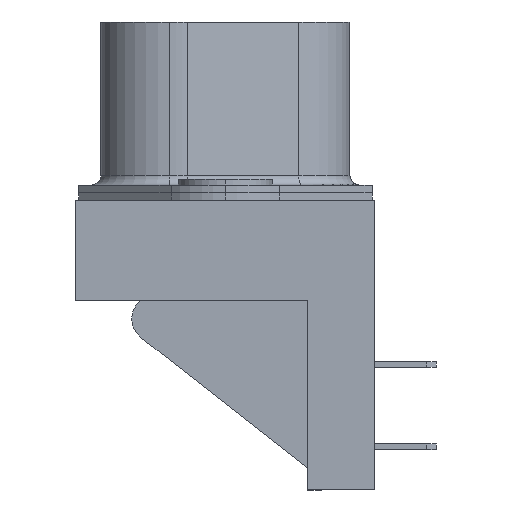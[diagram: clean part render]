
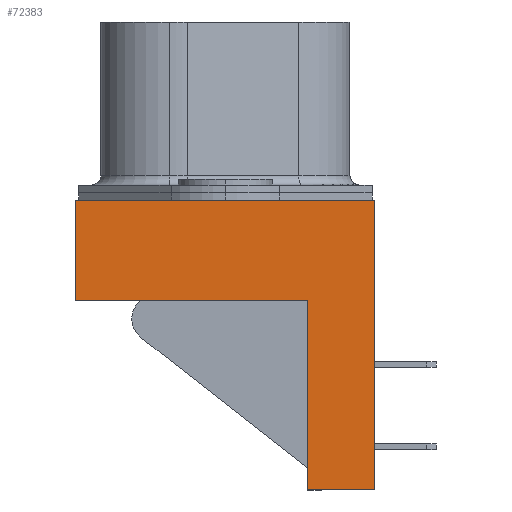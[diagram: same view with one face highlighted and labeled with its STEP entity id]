
A CAD part, left-side view. The second image highlights one B-rep face of the part: STEP entity #72383.
In plain terms, the highlighted planar face has unit normal (-1, 0, 0).
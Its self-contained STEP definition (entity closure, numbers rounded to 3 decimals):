
#6338 = VECTOR ( 'NONE', #7277, 1000. ) ;
#7079 = LINE ( 'NONE', #116483, #112464 ) ;
#7277 = DIRECTION ( 'NONE',  ( 0., 1., 0. ) ) ;
#9020 = CARTESIAN_POINT ( 'NONE',  ( -4.125, 7.8, -5.2 ) ) ;
#9100 = CARTESIAN_POINT ( 'NONE',  ( -4.125, 7.8, -15.1 ) ) ;
#12215 = ORIENTED_EDGE ( 'NONE', *, *, #30796, .T. ) ;
#16595 = EDGE_CURVE ( 'NONE', #127421, #80010, #158144, .T. ) ;
#17014 = AXIS2_PLACEMENT_3D ( 'NONE', #9100, #148927, #162362 ) ;
#20679 = CARTESIAN_POINT ( 'NONE',  ( -4.125, -7.8, -15.1 ) ) ;
#30796 = EDGE_CURVE ( 'NONE', #80010, #71657, #39707, .T. ) ;
#39707 = LINE ( 'NONE', #149103, #87490 ) ;
#47258 = DIRECTION ( 'NONE',  ( 0., 0., 1. ) ) ;
#51379 = DIRECTION ( 'NONE',  ( 0., 0., 1. ) ) ;
#57120 = EDGE_CURVE ( 'NONE', #147995, #71657, #125029, .T. ) ;
#58503 = VERTEX_POINT ( 'NONE', #109397 ) ;
#63355 = LINE ( 'NONE', #144104, #88697 ) ;
#64720 = VECTOR ( 'NONE', #99892, 1000. ) ;
#64874 = EDGE_CURVE ( 'NONE', #58503, #126019, #130157, .T. ) ;
#65377 = EDGE_CURVE ( 'NONE', #127421, #58503, #7079, .T. ) ;
#71657 = VERTEX_POINT ( 'NONE', #162786 ) ;
#72383 = ADVANCED_FACE ( 'NONE', ( #74632 ), #129359, .T. ) ;
#74632 = FACE_OUTER_BOUND ( 'NONE', #95636, .T. ) ;
#76342 = CARTESIAN_POINT ( 'NONE',  ( -4.125, 7.8, -5.2 ) ) ;
#80010 = VERTEX_POINT ( 'NONE', #20679 ) ;
#87490 = VECTOR ( 'NONE', #51379, 1000. ) ;
#88697 = VECTOR ( 'NONE', #47258, 1000. ) ;
#89996 = DIRECTION ( 'NONE',  ( 0., -1., 0. ) ) ;
#90868 = CARTESIAN_POINT ( 'NONE',  ( -4.125, 7.8, -15.1 ) ) ;
#93378 = EDGE_CURVE ( 'NONE', #126019, #147995, #63355, .T. ) ;
#95636 = EDGE_LOOP ( 'NONE', ( #129250, #99727, #172409, #12215, #135933, #114596 ) ) ;
#99727 = ORIENTED_EDGE ( 'NONE', *, *, #65377, .F. ) ;
#99892 = DIRECTION ( 'NONE',  ( 0., -1., 0. ) ) ;
#101210 = CARTESIAN_POINT ( 'NONE',  ( -4.125, 7.8, 0. ) ) ;
#109397 = CARTESIAN_POINT ( 'NONE',  ( -4.125, -4.3, -5.2 ) ) ;
#112464 = VECTOR ( 'NONE', #171159, 1000. ) ;
#114596 = ORIENTED_EDGE ( 'NONE', *, *, #93378, .F. ) ;
#116483 = CARTESIAN_POINT ( 'NONE',  ( -4.125, -4.3, -15.1 ) ) ;
#125029 = LINE ( 'NONE', #126829, #64720 ) ;
#126019 = VERTEX_POINT ( 'NONE', #76342 ) ;
#126829 = CARTESIAN_POINT ( 'NONE',  ( -4.125, 7.8, 0. ) ) ;
#127421 = VERTEX_POINT ( 'NONE', #143455 ) ;
#129250 = ORIENTED_EDGE ( 'NONE', *, *, #64874, .F. ) ;
#129359 = PLANE ( 'NONE',  #17014 ) ;
#130157 = LINE ( 'NONE', #9020, #6338 ) ;
#135933 = ORIENTED_EDGE ( 'NONE', *, *, #57120, .F. ) ;
#143455 = CARTESIAN_POINT ( 'NONE',  ( -4.125, -4.3, -15.1 ) ) ;
#144104 = CARTESIAN_POINT ( 'NONE',  ( -4.125, 7.8, -15.1 ) ) ;
#147995 = VERTEX_POINT ( 'NONE', #101210 ) ;
#148927 = DIRECTION ( 'NONE',  ( -1., 0., 0. ) ) ;
#149103 = CARTESIAN_POINT ( 'NONE',  ( -4.125, -7.8, -15.1 ) ) ;
#158144 = LINE ( 'NONE', #90868, #175677 ) ;
#162362 = DIRECTION ( 'NONE',  ( 0., -1., 0. ) ) ;
#162786 = CARTESIAN_POINT ( 'NONE',  ( -4.125, -7.8, 0. ) ) ;
#171159 = DIRECTION ( 'NONE',  ( 0., 0., 1. ) ) ;
#172409 = ORIENTED_EDGE ( 'NONE', *, *, #16595, .T. ) ;
#175677 = VECTOR ( 'NONE', #89996, 1000. ) ;
